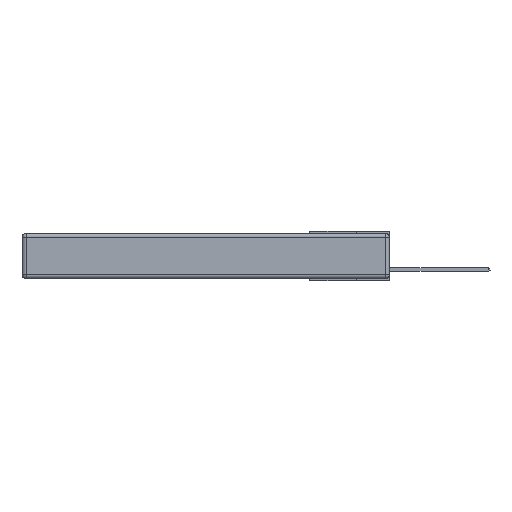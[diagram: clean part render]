
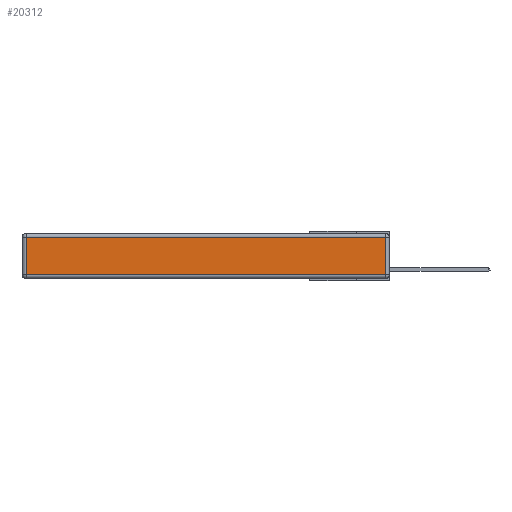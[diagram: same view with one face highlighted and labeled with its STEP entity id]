
A CAD part, left-side view. The second image highlights one B-rep face of the part: STEP entity #20312.
In plain terms, the highlighted planar face has unit normal (-1, 0, 0).
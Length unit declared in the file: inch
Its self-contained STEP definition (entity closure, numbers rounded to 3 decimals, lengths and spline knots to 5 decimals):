
#155 = VECTOR ( 'NONE', #14921, 39.37008 ) ;
#298 = VERTEX_POINT ( 'NONE', #5540 ) ;
#325 = FACE_OUTER_BOUND ( 'NONE', #14424, .T. ) ;
#664 = ORIENTED_EDGE ( 'NONE', *, *, #8589, .T. ) ;
#2968 = ORIENTED_EDGE ( 'NONE', *, *, #21122, .T. ) ;
#3188 = DIRECTION ( 'NONE',  ( 0., -1., 0. ) ) ;
#5540 = CARTESIAN_POINT ( 'NONE',  ( 0., 0.03, -0.313 ) ) ;
#8589 = EDGE_CURVE ( 'NONE', #20598, #28134, #12295, .T. ) ;
#8861 = DIRECTION ( 'NONE',  ( -1., 0., 0. ) ) ;
#9895 = VECTOR ( 'NONE', #24956, 39.37008 ) ;
#9951 = CARTESIAN_POINT ( 'NONE',  ( 0., 2.75, -0.03 ) ) ;
#10839 = CARTESIAN_POINT ( 'NONE',  ( 0., 0., -0.313 ) ) ;
#12112 = DIRECTION ( 'NONE',  ( 0., 0., 1. ) ) ;
#12295 = LINE ( 'NONE', #17089, #9895 ) ;
#14424 = EDGE_LOOP ( 'NONE', ( #31541, #2968, #19541, #664 ) ) ;
#14613 = CARTESIAN_POINT ( 'NONE',  ( 0., 2.72, -0.313 ) ) ;
#14737 = CARTESIAN_POINT ( 'NONE',  ( 0., 0.03, -0.343 ) ) ;
#14921 = DIRECTION ( 'NONE',  ( 0., 1., 0. ) ) ;
#15452 = CARTESIAN_POINT ( 'NONE',  ( 0., 2.72, -0.03 ) ) ;
#17089 = CARTESIAN_POINT ( 'NONE',  ( 0., 2.72, -0.343 ) ) ;
#18926 = PLANE ( 'NONE',  #26551 ) ;
#19541 = ORIENTED_EDGE ( 'NONE', *, *, #25611, .T. ) ;
#19706 = LINE ( 'NONE', #10839, #31569 ) ;
#19923 = CARTESIAN_POINT ( 'NONE',  ( 0., 0.03, -0.03 ) ) ;
#20312 = ADVANCED_FACE ( 'NONE', ( #325 ), #18926, .T. ) ;
#20598 = VERTEX_POINT ( 'NONE', #15452 ) ;
#20617 = EDGE_CURVE ( 'NONE', #28134, #298, #19706, .T. ) ;
#21122 = EDGE_CURVE ( 'NONE', #298, #26853, #22068, .T. ) ;
#21958 = LINE ( 'NONE', #9951, #155 ) ;
#22068 = LINE ( 'NONE', #14737, #31148 ) ;
#24039 = CARTESIAN_POINT ( 'NONE',  ( 0., 0., -0.343 ) ) ;
#24956 = DIRECTION ( 'NONE',  ( 0., 0., -1. ) ) ;
#25611 = EDGE_CURVE ( 'NONE', #26853, #20598, #21958, .T. ) ;
#26551 = AXIS2_PLACEMENT_3D ( 'NONE', #24039, #8861, #26577 ) ;
#26577 = DIRECTION ( 'NONE',  ( 0., 0., 1. ) ) ;
#26853 = VERTEX_POINT ( 'NONE', #19923 ) ;
#28134 = VERTEX_POINT ( 'NONE', #14613 ) ;
#31148 = VECTOR ( 'NONE', #12112, 39.37008 ) ;
#31541 = ORIENTED_EDGE ( 'NONE', *, *, #20617, .T. ) ;
#31569 = VECTOR ( 'NONE', #3188, 39.37008 ) ;
